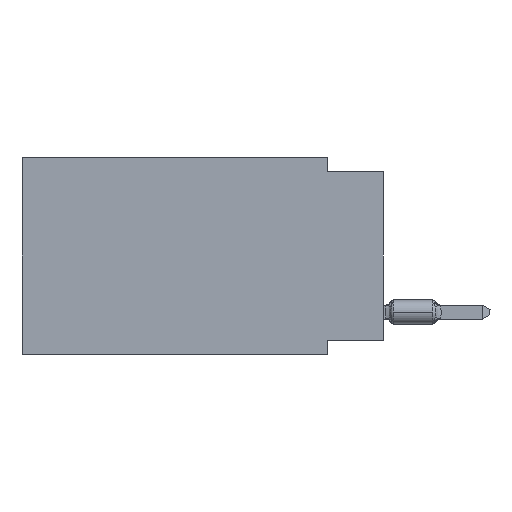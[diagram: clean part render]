
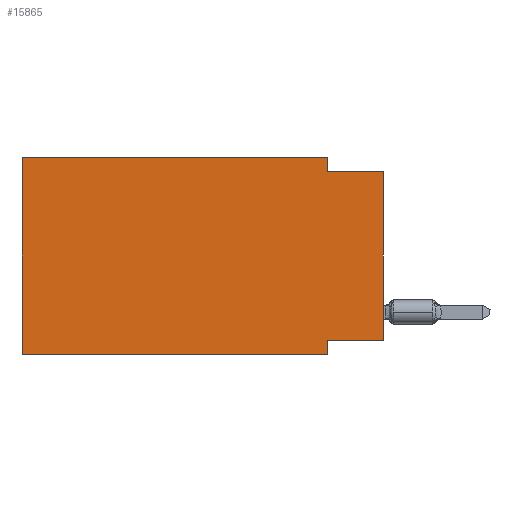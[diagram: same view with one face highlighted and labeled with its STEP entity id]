
A CAD part, left-side view. The second image highlights one B-rep face of the part: STEP entity #15865.
In plain terms, the highlighted planar face has unit normal (-1, 0, 0).
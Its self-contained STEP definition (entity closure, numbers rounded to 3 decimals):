
#179 = CARTESIAN_POINT ( 'NONE',  ( 0., 0., -0.635 ) ) ;
#1143 = VERTEX_POINT ( 'NONE', #7588 ) ;
#1157 = EDGE_CURVE ( 'NONE', #7655, #24840, #17563, .T. ) ;
#1948 = DIRECTION ( 'NONE',  ( 0., 0., -1. ) ) ;
#1961 = DIRECTION ( 'NONE',  ( 0., -1., 0. ) ) ;
#2391 = CARTESIAN_POINT ( 'NONE',  ( 0., 16.383, -8.89 ) ) ;
#3509 = CARTESIAN_POINT ( 'NONE',  ( 0., 0., 0. ) ) ;
#3954 = ORIENTED_EDGE ( 'NONE', *, *, #5218, .F. ) ;
#4970 = CARTESIAN_POINT ( 'NONE',  ( 0., 16.383, 0. ) ) ;
#5218 = EDGE_CURVE ( 'NONE', #22086, #1143, #11768, .T. ) ;
#5689 = EDGE_CURVE ( 'NONE', #24840, #36596, #26177, .T. ) ;
#6053 = CARTESIAN_POINT ( 'NONE',  ( 0., 2.54, 0. ) ) ;
#7588 = CARTESIAN_POINT ( 'NONE',  ( 0., 2.54, -8.255 ) ) ;
#7655 = VERTEX_POINT ( 'NONE', #6053 ) ;
#8029 = ORIENTED_EDGE ( 'NONE', *, *, #1157, .F. ) ;
#8925 = DIRECTION ( 'NONE',  ( 0., 0., -1. ) ) ;
#9082 = ORIENTED_EDGE ( 'NONE', *, *, #12446, .T. ) ;
#9615 = AXIS2_PLACEMENT_3D ( 'NONE', #31029, #11516, #8925 ) ;
#11221 = VECTOR ( 'NONE', #16737, 1000. ) ;
#11257 = CARTESIAN_POINT ( 'NONE',  ( 0., 2.54, 0. ) ) ;
#11516 = DIRECTION ( 'NONE',  ( 1., 0., 0. ) ) ;
#11768 = LINE ( 'NONE', #31068, #38459 ) ;
#11772 = LINE ( 'NONE', #31512, #30240 ) ;
#12446 = EDGE_CURVE ( 'NONE', #22086, #36596, #33203, .T. ) ;
#13077 = VERTEX_POINT ( 'NONE', #31394 ) ;
#13288 = CARTESIAN_POINT ( 'NONE',  ( 0., 0., -8.255 ) ) ;
#13968 = ORIENTED_EDGE ( 'NONE', *, *, #5689, .F. ) ;
#14252 = ORIENTED_EDGE ( 'NONE', *, *, #25248, .T. ) ;
#15865 = ADVANCED_FACE ( 'NONE', ( #18685 ), #37750, .F. ) ;
#16737 = DIRECTION ( 'NONE',  ( 0., 0., 1. ) ) ;
#17404 = CARTESIAN_POINT ( 'NONE',  ( 0., 0., -0.635 ) ) ;
#17563 = LINE ( 'NONE', #11257, #17848 ) ;
#17848 = VECTOR ( 'NONE', #24481, 1000. ) ;
#18167 = ORIENTED_EDGE ( 'NONE', *, *, #25040, .F. ) ;
#18685 = FACE_OUTER_BOUND ( 'NONE', #35484, .T. ) ;
#19501 = CARTESIAN_POINT ( 'NONE',  ( 0., 2.54, -8.89 ) ) ;
#22086 = VERTEX_POINT ( 'NONE', #13288 ) ;
#24481 = DIRECTION ( 'NONE',  ( 0., 0., -1. ) ) ;
#24840 = VERTEX_POINT ( 'NONE', #42006 ) ;
#25040 = EDGE_CURVE ( 'NONE', #1143, #32169, #41842, .T. ) ;
#25248 = EDGE_CURVE ( 'NONE', #41370, #32169, #42691, .T. ) ;
#25310 = ORIENTED_EDGE ( 'NONE', *, *, #26402, .F. ) ;
#26177 = LINE ( 'NONE', #179, #34347 ) ;
#26402 = EDGE_CURVE ( 'NONE', #41370, #13077, #37691, .T. ) ;
#28289 = EDGE_CURVE ( 'NONE', #13077, #7655, #11772, .T. ) ;
#30240 = VECTOR ( 'NONE', #38224, 1000. ) ;
#30453 = VECTOR ( 'NONE', #1948, 1000. ) ;
#31029 = CARTESIAN_POINT ( 'NONE',  ( 0., 16.383, 0. ) ) ;
#31068 = CARTESIAN_POINT ( 'NONE',  ( 0., 0., -8.255 ) ) ;
#31394 = CARTESIAN_POINT ( 'NONE',  ( 0., 16.383, 0. ) ) ;
#31512 = CARTESIAN_POINT ( 'NONE',  ( 0., 16.383, 0. ) ) ;
#32169 = VERTEX_POINT ( 'NONE', #19501 ) ;
#33203 = LINE ( 'NONE', #3509, #11221 ) ;
#34036 = DIRECTION ( 'NONE',  ( 0., 0., 1. ) ) ;
#34347 = VECTOR ( 'NONE', #1961, 1000. ) ;
#34758 = DIRECTION ( 'NONE',  ( 0., 1., 0. ) ) ;
#35120 = CARTESIAN_POINT ( 'NONE',  ( 0., 2.54, -8.89 ) ) ;
#35484 = EDGE_LOOP ( 'NONE', ( #9082, #13968, #8029, #40347, #25310, #14252, #18167, #3954 ) ) ;
#36196 = DIRECTION ( 'NONE',  ( 0., -1., 0. ) ) ;
#36596 = VERTEX_POINT ( 'NONE', #17404 ) ;
#37691 = LINE ( 'NONE', #4970, #41612 ) ;
#37750 = PLANE ( 'NONE',  #9615 ) ;
#38061 = VECTOR ( 'NONE', #36196, 1000. ) ;
#38224 = DIRECTION ( 'NONE',  ( 0., -1., 0. ) ) ;
#38459 = VECTOR ( 'NONE', #34758, 1000. ) ;
#39471 = CARTESIAN_POINT ( 'NONE',  ( 0., 16.383, -8.89 ) ) ;
#40347 = ORIENTED_EDGE ( 'NONE', *, *, #28289, .F. ) ;
#41370 = VERTEX_POINT ( 'NONE', #39471 ) ;
#41612 = VECTOR ( 'NONE', #34036, 1000. ) ;
#41842 = LINE ( 'NONE', #35120, #30453 ) ;
#42006 = CARTESIAN_POINT ( 'NONE',  ( 0., 2.54, -0.635 ) ) ;
#42691 = LINE ( 'NONE', #2391, #38061 ) ;
